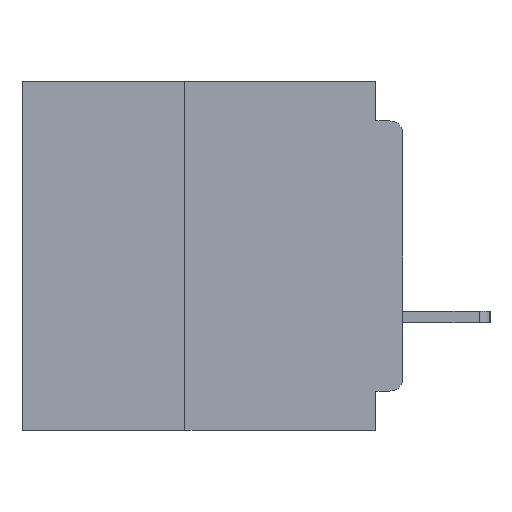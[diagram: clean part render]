
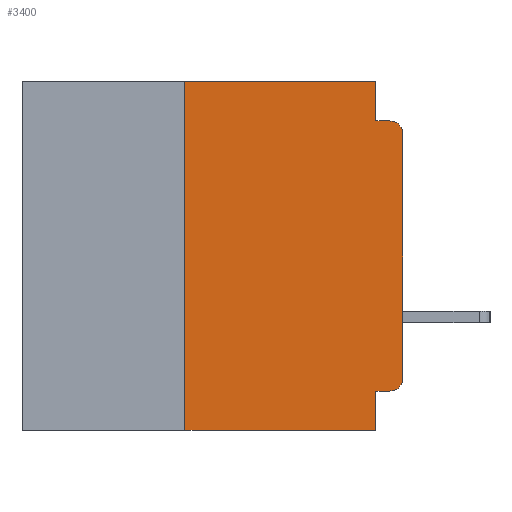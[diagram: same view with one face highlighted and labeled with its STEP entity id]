
A CAD part, left-side view. The second image highlights one B-rep face of the part: STEP entity #3400.
In plain terms, the highlighted planar face has unit normal (-1, 0, 0).
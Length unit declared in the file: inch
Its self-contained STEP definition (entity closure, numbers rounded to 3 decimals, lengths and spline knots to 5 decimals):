
#11 = EDGE_CURVE ( 'NONE', #8110, #27857, #36780, .T. ) ;
#355 = VECTOR ( 'NONE', #24661, 39.37008 ) ;
#951 = DIRECTION ( 'NONE',  ( -1., 0., 0. ) ) ;
#1097 = EDGE_CURVE ( 'NONE', #10324, #27669, #15282, .T. ) ;
#1766 = CARTESIAN_POINT ( 'NONE',  ( 0., 0.25, -0.4 ) ) ;
#2522 = DIRECTION ( 'NONE',  ( 0., 1., 0. ) ) ;
#3400 = ADVANCED_FACE ( 'NONE', ( #26574 ), #11120, .F. ) ;
#3557 = ORIENTED_EDGE ( 'NONE', *, *, #19489, .T. ) ;
#3618 = ORIENTED_EDGE ( 'NONE', *, *, #30825, .T. ) ;
#3772 = CARTESIAN_POINT ( 'NONE',  ( 0., 0.015, -0.045 ) ) ;
#4513 = CARTESIAN_POINT ( 'NONE',  ( 0., 0.015, -0.355 ) ) ;
#4543 = CARTESIAN_POINT ( 'NONE',  ( 0., 0., 0. ) ) ;
#4616 = VERTEX_POINT ( 'NONE', #3772 ) ;
#5201 = VERTEX_POINT ( 'NONE', #10235 ) ;
#5709 = VECTOR ( 'NONE', #14220, 39.37008 ) ;
#8110 = VERTEX_POINT ( 'NONE', #1766 ) ;
#8192 = LINE ( 'NONE', #13986, #28407 ) ;
#9153 = DIRECTION ( 'NONE',  ( 0., -1., 0. ) ) ;
#9593 = EDGE_CURVE ( 'NONE', #20796, #4616, #31575, .T. ) ;
#9884 = EDGE_CURVE ( 'NONE', #34362, #5201, #21733, .T. ) ;
#10185 = ORIENTED_EDGE ( 'NONE', *, *, #9593, .F. ) ;
#10235 = CARTESIAN_POINT ( 'NONE',  ( 0., 0., -0.34 ) ) ;
#10324 = VERTEX_POINT ( 'NONE', #23800 ) ;
#10968 = DIRECTION ( 'NONE',  ( 0., 0., -1. ) ) ;
#11006 = DIRECTION ( 'NONE',  ( 1., 0., 0. ) ) ;
#11020 = VERTEX_POINT ( 'NONE', #18882 ) ;
#11097 = CARTESIAN_POINT ( 'NONE',  ( 0., 0.437, 0. ) ) ;
#11120 = PLANE ( 'NONE',  #18427 ) ;
#11219 = CARTESIAN_POINT ( 'NONE',  ( 0., 0., -0.045 ) ) ;
#11280 = CARTESIAN_POINT ( 'NONE',  ( 0., 0., -0.06 ) ) ;
#11505 = DIRECTION ( 'NONE',  ( 0., -1., 0. ) ) ;
#13192 = EDGE_CURVE ( 'NONE', #27857, #11020, #37022, .T. ) ;
#13356 = VECTOR ( 'NONE', #11505, 39.37008 ) ;
#13427 = CARTESIAN_POINT ( 'NONE',  ( 0., 0.25, -0.4 ) ) ;
#13986 = CARTESIAN_POINT ( 'NONE',  ( 0., 0., -0.355 ) ) ;
#14220 = DIRECTION ( 'NONE',  ( 0., 0., -1. ) ) ;
#14626 = EDGE_LOOP ( 'NONE', ( #17223, #3557, #10185, #33300, #26135, #27300, #3618, #30817, #26257, #26403 ) ) ;
#14799 = DIRECTION ( 'NONE',  ( 0., 0., 1. ) ) ;
#14920 = VECTOR ( 'NONE', #14799, 39.37008 ) ;
#15282 = LINE ( 'NONE', #16224, #30507 ) ;
#15451 = EDGE_CURVE ( 'NONE', #5201, #15690, #30882, .T. ) ;
#15496 = DIRECTION ( 'NONE',  ( -1., 0., 0. ) ) ;
#15660 = DIRECTION ( 'NONE',  ( 0., 0., -1. ) ) ;
#15690 = VERTEX_POINT ( 'NONE', #11280 ) ;
#16164 = EDGE_CURVE ( 'NONE', #11020, #20796, #28587, .T. ) ;
#16224 = CARTESIAN_POINT ( 'NONE',  ( 0., 0.031, -0.4 ) ) ;
#17112 = CARTESIAN_POINT ( 'NONE',  ( 0., 0.031, 0. ) ) ;
#17223 = ORIENTED_EDGE ( 'NONE', *, *, #15451, .T. ) ;
#17333 = CARTESIAN_POINT ( 'NONE',  ( 0., 0.437, 0. ) ) ;
#17648 = CARTESIAN_POINT ( 'NONE',  ( 0., 0.031, -0.4 ) ) ;
#17763 = CARTESIAN_POINT ( 'NONE',  ( 0., 0.437, -0.4 ) ) ;
#18208 = CARTESIAN_POINT ( 'NONE',  ( 0., 0.015, -0.06 ) ) ;
#18427 = AXIS2_PLACEMENT_3D ( 'NONE', #11097, #11006, #10968 ) ;
#18882 = CARTESIAN_POINT ( 'NONE',  ( 0., 0.031, 0. ) ) ;
#19489 = EDGE_CURVE ( 'NONE', #15690, #4616, #33277, .T. ) ;
#19862 = AXIS2_PLACEMENT_3D ( 'NONE', #18208, #951, #21081 ) ;
#20796 = VERTEX_POINT ( 'NONE', #24143 ) ;
#21081 = DIRECTION ( 'NONE',  ( 0., 0., -1. ) ) ;
#21733 = CIRCLE ( 'NONE', #24575, 0.015 ) ;
#23800 = CARTESIAN_POINT ( 'NONE',  ( 0., 0.031, -0.355 ) ) ;
#24014 = VECTOR ( 'NONE', #36956, 39.37008 ) ;
#24143 = CARTESIAN_POINT ( 'NONE',  ( 0., 0.031, -0.045 ) ) ;
#24419 = CARTESIAN_POINT ( 'NONE',  ( 0., 0.25, 0. ) ) ;
#24575 = AXIS2_PLACEMENT_3D ( 'NONE', #32657, #15496, #35461 ) ;
#24661 = DIRECTION ( 'NONE',  ( 0., 0., 1. ) ) ;
#26135 = ORIENTED_EDGE ( 'NONE', *, *, #13192, .F. ) ;
#26257 = ORIENTED_EDGE ( 'NONE', *, *, #29352, .F. ) ;
#26403 = ORIENTED_EDGE ( 'NONE', *, *, #9884, .T. ) ;
#26574 = FACE_OUTER_BOUND ( 'NONE', #14626, .T. ) ;
#27300 = ORIENTED_EDGE ( 'NONE', *, *, #11, .F. ) ;
#27669 = VERTEX_POINT ( 'NONE', #17648 ) ;
#27857 = VERTEX_POINT ( 'NONE', #24419 ) ;
#28407 = VECTOR ( 'NONE', #2522, 39.37008 ) ;
#28587 = LINE ( 'NONE', #17112, #5709 ) ;
#28732 = LINE ( 'NONE', #17763, #35383 ) ;
#29352 = EDGE_CURVE ( 'NONE', #34362, #10324, #8192, .T. ) ;
#30507 = VECTOR ( 'NONE', #15660, 39.37008 ) ;
#30817 = ORIENTED_EDGE ( 'NONE', *, *, #1097, .F. ) ;
#30825 = EDGE_CURVE ( 'NONE', #8110, #27669, #28732, .T. ) ;
#30882 = LINE ( 'NONE', #4543, #355 ) ;
#31575 = LINE ( 'NONE', #11219, #24014 ) ;
#32657 = CARTESIAN_POINT ( 'NONE',  ( 0., 0.015, -0.34 ) ) ;
#33277 = CIRCLE ( 'NONE', #19862, 0.015 ) ;
#33300 = ORIENTED_EDGE ( 'NONE', *, *, #16164, .F. ) ;
#34362 = VERTEX_POINT ( 'NONE', #4513 ) ;
#35383 = VECTOR ( 'NONE', #9153, 39.37008 ) ;
#35461 = DIRECTION ( 'NONE',  ( 0., 0., -1. ) ) ;
#36780 = LINE ( 'NONE', #13427, #14920 ) ;
#36956 = DIRECTION ( 'NONE',  ( 0., -1., 0. ) ) ;
#37022 = LINE ( 'NONE', #17333, #13356 ) ;
